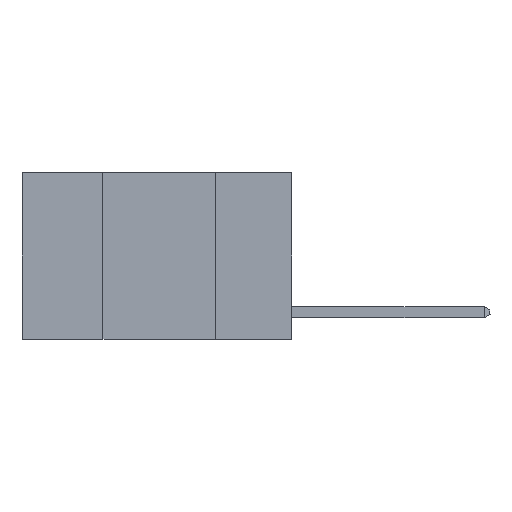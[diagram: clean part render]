
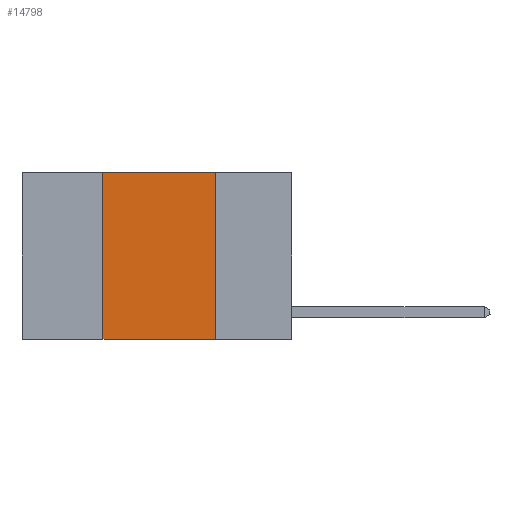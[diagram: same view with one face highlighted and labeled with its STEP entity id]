
A CAD part, left-side view. The second image highlights one B-rep face of the part: STEP entity #14798.
In plain terms, the highlighted planar face has unit normal (-1, 0, 0).
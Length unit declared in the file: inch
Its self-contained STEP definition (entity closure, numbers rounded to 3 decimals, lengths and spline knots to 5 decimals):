
#25 = VECTOR ( 'NONE', #4163, 39.37008 ) ;
#1750 = DIRECTION ( 'NONE',  ( 0., 0., 1. ) ) ;
#2110 = VERTEX_POINT ( 'NONE', #10503 ) ;
#2289 = PLANE ( 'NONE',  #14308 ) ;
#2418 = CARTESIAN_POINT ( 'NONE',  ( 0., 0.42, -0.37 ) ) ;
#3779 = EDGE_CURVE ( 'NONE', #25101, #5105, #22601, .T. ) ;
#4163 = DIRECTION ( 'NONE',  ( 0., -1., 0. ) ) ;
#4174 = VECTOR ( 'NONE', #25615, 39.37008 ) ;
#4297 = DIRECTION ( 'NONE',  ( 0., 0., -1. ) ) ;
#5105 = VERTEX_POINT ( 'NONE', #22253 ) ;
#5312 = EDGE_LOOP ( 'NONE', ( #6415, #12342, #19157, #12366 ) ) ;
#6142 = CARTESIAN_POINT ( 'NONE',  ( 0., 0.6, 0. ) ) ;
#6415 = ORIENTED_EDGE ( 'NONE', *, *, #20075, .F. ) ;
#8584 = VECTOR ( 'NONE', #9102, 39.37008 ) ;
#9102 = DIRECTION ( 'NONE',  ( 0., 0., -1. ) ) ;
#9673 = CARTESIAN_POINT ( 'NONE',  ( 0., 0.42, 0. ) ) ;
#10238 = FACE_OUTER_BOUND ( 'NONE', #5312, .T. ) ;
#10503 = CARTESIAN_POINT ( 'NONE',  ( 0., 0.17, 0. ) ) ;
#12342 = ORIENTED_EDGE ( 'NONE', *, *, #22027, .F. ) ;
#12366 = ORIENTED_EDGE ( 'NONE', *, *, #20699, .T. ) ;
#13746 = CARTESIAN_POINT ( 'NONE',  ( 0., 0.6, -0.37 ) ) ;
#13821 = LINE ( 'NONE', #22950, #8584 ) ;
#14308 = AXIS2_PLACEMENT_3D ( 'NONE', #24051, #16170, #4297 ) ;
#14798 = ADVANCED_FACE ( 'NONE', ( #10238 ), #2289, .F. ) ;
#15317 = LINE ( 'NONE', #13746, #4174 ) ;
#16080 = VECTOR ( 'NONE', #1750, 39.37008 ) ;
#16170 = DIRECTION ( 'NONE',  ( 1., 0., 0. ) ) ;
#19157 = ORIENTED_EDGE ( 'NONE', *, *, #3779, .F. ) ;
#20075 = EDGE_CURVE ( 'NONE', #2110, #25297, #13821, .T. ) ;
#20544 = LINE ( 'NONE', #6142, #25 ) ;
#20699 = EDGE_CURVE ( 'NONE', #25101, #25297, #15317, .T. ) ;
#20868 = CARTESIAN_POINT ( 'NONE',  ( 0., 0.17, -0.37 ) ) ;
#22027 = EDGE_CURVE ( 'NONE', #5105, #2110, #20544, .T. ) ;
#22253 = CARTESIAN_POINT ( 'NONE',  ( 0., 0.42, 0. ) ) ;
#22601 = LINE ( 'NONE', #9673, #16080 ) ;
#22950 = CARTESIAN_POINT ( 'NONE',  ( 0., 0.17, 0. ) ) ;
#24051 = CARTESIAN_POINT ( 'NONE',  ( 0., 0.6, 0. ) ) ;
#25101 = VERTEX_POINT ( 'NONE', #2418 ) ;
#25297 = VERTEX_POINT ( 'NONE', #20868 ) ;
#25615 = DIRECTION ( 'NONE',  ( 0., -1., 0. ) ) ;
